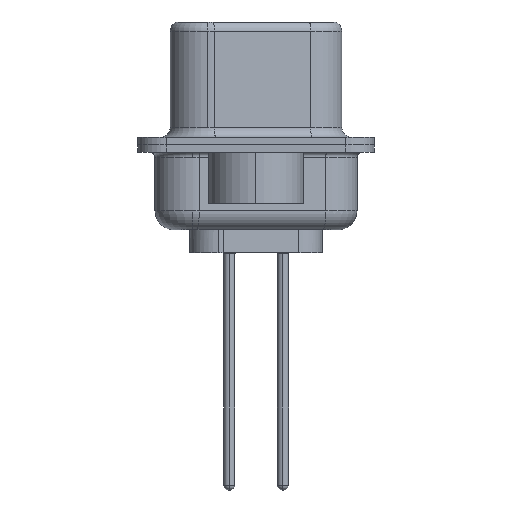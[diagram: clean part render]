
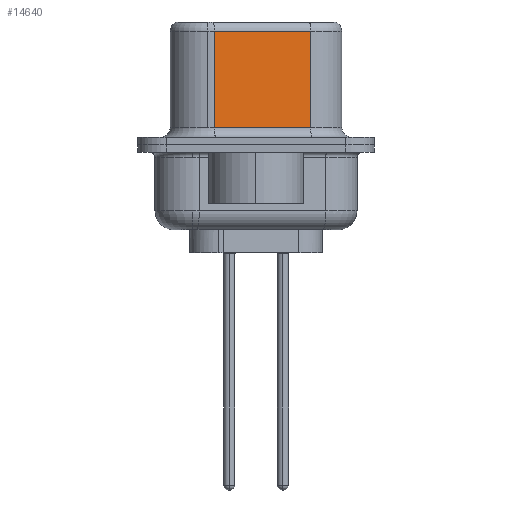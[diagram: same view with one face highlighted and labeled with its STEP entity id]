
A CAD part, left-side view. The second image highlights one B-rep face of the part: STEP entity #14640.
In plain terms, the highlighted planar face has unit normal (-0.985, -0.174, 0).
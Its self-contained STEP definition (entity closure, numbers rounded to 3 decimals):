
#186 = CARTESIAN_POINT ( 'NONE',  ( 4.58, -2.897, 0.9 ) ) ;
#909 = DIRECTION ( 'NONE',  ( 0.985, 0.174, 0. ) ) ;
#2524 = CARTESIAN_POINT ( 'NONE',  ( 3.68, 2.203, 6.02 ) ) ;
#2670 = ORIENTED_EDGE ( 'NONE', *, *, #8788, .T. ) ;
#2678 = EDGE_CURVE ( 'NONE', #7104, #14341, #13486, .T. ) ;
#2963 = VECTOR ( 'NONE', #19870, 1000. ) ;
#3860 = FACE_OUTER_BOUND ( 'NONE', #4716, .T. ) ;
#4716 = EDGE_LOOP ( 'NONE', ( #16398, #12483, #17599, #2670 ) ) ;
#4751 = VERTEX_POINT ( 'NONE', #2524 ) ;
#5639 = LINE ( 'NONE', #12143, #15479 ) ;
#7104 = VERTEX_POINT ( 'NONE', #13477 ) ;
#7693 = DIRECTION ( 'NONE',  ( -0.174, 0.985, 0. ) ) ;
#8419 = VECTOR ( 'NONE', #7693, 1000. ) ;
#8652 = DIRECTION ( 'NONE',  ( -0.174, 0.985, 0. ) ) ;
#8788 = EDGE_CURVE ( 'NONE', #12240, #14341, #14486, .T. ) ;
#9452 = CARTESIAN_POINT ( 'NONE',  ( 4.58, -2.897, 0.9 ) ) ;
#9726 = VECTOR ( 'NONE', #15846, 1000. ) ;
#10031 = EDGE_CURVE ( 'NONE', #7104, #4751, #10854, .T. ) ;
#10238 = PLANE ( 'NONE',  #17571 ) ;
#10854 = LINE ( 'NONE', #15672, #8419 ) ;
#11687 = CARTESIAN_POINT ( 'NONE',  ( 4.58, -2.897, 6.52 ) ) ;
#12143 = CARTESIAN_POINT ( 'NONE',  ( 3.68, 2.203, 6.52 ) ) ;
#12240 = VERTEX_POINT ( 'NONE', #16373 ) ;
#12483 = ORIENTED_EDGE ( 'NONE', *, *, #10031, .T. ) ;
#13477 = CARTESIAN_POINT ( 'NONE',  ( 4.58, -2.897, 6.02 ) ) ;
#13486 = LINE ( 'NONE', #11687, #2963 ) ;
#14341 = VERTEX_POINT ( 'NONE', #186 ) ;
#14486 = LINE ( 'NONE', #9452, #9726 ) ;
#14640 = ADVANCED_FACE ( 'NONE', ( #3860 ), #10238, .F. ) ;
#15479 = VECTOR ( 'NONE', #18530, 1000. ) ;
#15672 = CARTESIAN_POINT ( 'NONE',  ( 4.58, -2.897, 6.02 ) ) ;
#15846 = DIRECTION ( 'NONE',  ( 0.174, -0.985, 0. ) ) ;
#16373 = CARTESIAN_POINT ( 'NONE',  ( 3.68, 2.203, 0.9 ) ) ;
#16398 = ORIENTED_EDGE ( 'NONE', *, *, #2678, .F. ) ;
#16624 = CARTESIAN_POINT ( 'NONE',  ( 4.58, -2.897, 6.52 ) ) ;
#17571 = AXIS2_PLACEMENT_3D ( 'NONE', #16624, #909, #8652 ) ;
#17599 = ORIENTED_EDGE ( 'NONE', *, *, #19968, .T. ) ;
#18530 = DIRECTION ( 'NONE',  ( 0., 0., -1. ) ) ;
#19870 = DIRECTION ( 'NONE',  ( 0., 0., -1. ) ) ;
#19968 = EDGE_CURVE ( 'NONE', #4751, #12240, #5639, .T. ) ;
